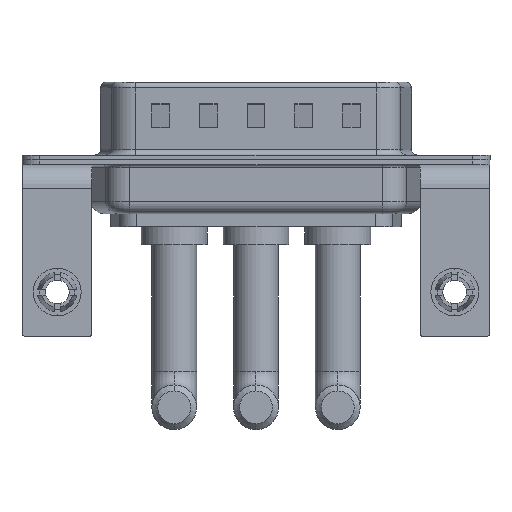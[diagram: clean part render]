
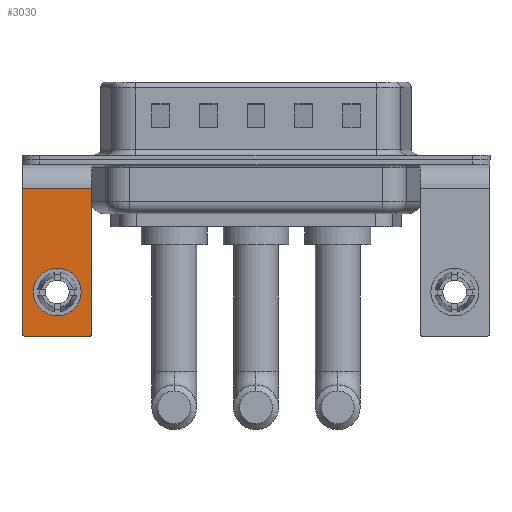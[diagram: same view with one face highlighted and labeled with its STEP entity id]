
A CAD part, front view. The second image highlights one B-rep face of the part: STEP entity #3030.
In plain terms, the highlighted planar face has unit normal (0, -1, 0).
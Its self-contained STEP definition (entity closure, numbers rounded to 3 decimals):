
#278 = EDGE_CURVE ( 'NONE', #8263, #9243, #16908, .T. ) ;
#371 = LINE ( 'NONE', #4820, #7940 ) ;
#404 = AXIS2_PLACEMENT_3D ( 'NONE', #13075, #552, #7573 ) ;
#552 = DIRECTION ( 'NONE',  ( 0., 1., 0. ) ) ;
#1110 = ORIENTED_EDGE ( 'NONE', *, *, #10544, .F. ) ;
#1682 = VERTEX_POINT ( 'NONE', #12028 ) ;
#1936 = VERTEX_POINT ( 'NONE', #9993 ) ;
#2019 = EDGE_LOOP ( 'NONE', ( #11203, #3994, #1110, #11894, #14713, #11677 ) ) ;
#2420 = EDGE_CURVE ( 'NONE', #9901, #11657, #15220, .T. ) ;
#3030 = ADVANCED_FACE ( 'NONE', ( #12803, #15634 ), #11686, .F. ) ;
#3065 = VECTOR ( 'NONE', #7328, 1000. ) ;
#3817 = EDGE_CURVE ( 'NONE', #1682, #9901, #5685, .T. ) ;
#3994 = ORIENTED_EDGE ( 'NONE', *, *, #2420, .T. ) ;
#4219 = CIRCLE ( 'NONE', #16773, 2. ) ;
#4284 = EDGE_CURVE ( 'NONE', #5242, #1682, #14102, .T. ) ;
#4475 = DIRECTION ( 'NONE',  ( 0., 0., 1. ) ) ;
#4621 = VERTEX_POINT ( 'NONE', #6673 ) ;
#4820 = CARTESIAN_POINT ( 'NONE',  ( 2.9, -6.25, -2.4 ) ) ;
#4847 = DIRECTION ( 'NONE',  ( 0., 0., 1. ) ) ;
#5165 = EDGE_CURVE ( 'NONE', #1936, #4621, #4219, .T. ) ;
#5186 = CIRCLE ( 'NONE', #11595, 2. ) ;
#5242 = VERTEX_POINT ( 'NONE', #13125 ) ;
#5439 = CARTESIAN_POINT ( 'NONE',  ( 2.9, -6.25, -14.8 ) ) ;
#5560 = AXIS2_PLACEMENT_3D ( 'NONE', #5772, #5858, #13947 ) ;
#5685 = LINE ( 'NONE', #11260, #3065 ) ;
#5772 = CARTESIAN_POINT ( 'NONE',  ( -2.65, -6.25, -14.55 ) ) ;
#5858 = DIRECTION ( 'NONE',  ( 0., -1., 0. ) ) ;
#6673 = CARTESIAN_POINT ( 'NONE',  ( 0., -6.25, -9.07 ) ) ;
#6827 = DIRECTION ( 'NONE',  ( 0., 1., 0. ) ) ;
#7141 = CARTESIAN_POINT ( 'NONE',  ( 2.9, -6.25, -14.55 ) ) ;
#7328 = DIRECTION ( 'NONE',  ( 0., 0., -1. ) ) ;
#7562 = DIRECTION ( 'NONE',  ( 0., 0., -1. ) ) ;
#7573 = DIRECTION ( 'NONE',  ( 0., 0., 1. ) ) ;
#7940 = VECTOR ( 'NONE', #7562, 1000. ) ;
#8263 = VERTEX_POINT ( 'NONE', #15278 ) ;
#8397 = EDGE_CURVE ( 'NONE', #5242, #9243, #371, .T. ) ;
#8854 = CARTESIAN_POINT ( 'NONE',  ( 0., -6.25, -11.07 ) ) ;
#9010 = AXIS2_PLACEMENT_3D ( 'NONE', #16006, #13374, #4847 ) ;
#9243 = VERTEX_POINT ( 'NONE', #7141 ) ;
#9555 = CARTESIAN_POINT ( 'NONE',  ( 0., -6.25, -11.07 ) ) ;
#9901 = VERTEX_POINT ( 'NONE', #10209 ) ;
#9993 = CARTESIAN_POINT ( 'NONE',  ( 0., -6.25, -13.07 ) ) ;
#10209 = CARTESIAN_POINT ( 'NONE',  ( -2.9, -6.25, -14.55 ) ) ;
#10544 = EDGE_CURVE ( 'NONE', #8263, #11657, #12570, .T. ) ;
#10615 = ORIENTED_EDGE ( 'NONE', *, *, #5165, .T. ) ;
#10754 = VECTOR ( 'NONE', #11234, 1000. ) ;
#10917 = VECTOR ( 'NONE', #18078, 1000. ) ;
#11203 = ORIENTED_EDGE ( 'NONE', *, *, #3817, .T. ) ;
#11234 = DIRECTION ( 'NONE',  ( -1., 0., 0. ) ) ;
#11260 = CARTESIAN_POINT ( 'NONE',  ( -2.9, -6.25, -2.4 ) ) ;
#11595 = AXIS2_PLACEMENT_3D ( 'NONE', #8854, #12978, #4475 ) ;
#11657 = VERTEX_POINT ( 'NONE', #15060 ) ;
#11677 = ORIENTED_EDGE ( 'NONE', *, *, #4284, .T. ) ;
#11686 = PLANE ( 'NONE',  #404 ) ;
#11894 = ORIENTED_EDGE ( 'NONE', *, *, #278, .T. ) ;
#12028 = CARTESIAN_POINT ( 'NONE',  ( -2.9, -6.25, -2.4 ) ) ;
#12570 = LINE ( 'NONE', #5439, #10917 ) ;
#12803 = FACE_BOUND ( 'NONE', #15481, .T. ) ;
#12978 = DIRECTION ( 'NONE',  ( 0., 1., 0. ) ) ;
#13075 = CARTESIAN_POINT ( 'NONE',  ( 2.9, -6.25, -2.4 ) ) ;
#13125 = CARTESIAN_POINT ( 'NONE',  ( 2.9, -6.25, -2.4 ) ) ;
#13374 = DIRECTION ( 'NONE',  ( 0., -1., 0. ) ) ;
#13947 = DIRECTION ( 'NONE',  ( 0., 0., 1. ) ) ;
#14102 = LINE ( 'NONE', #14280, #10754 ) ;
#14280 = CARTESIAN_POINT ( 'NONE',  ( 2.9, -6.25, -2.4 ) ) ;
#14713 = ORIENTED_EDGE ( 'NONE', *, *, #8397, .F. ) ;
#15060 = CARTESIAN_POINT ( 'NONE',  ( -2.65, -6.25, -14.8 ) ) ;
#15163 = DIRECTION ( 'NONE',  ( 0., 0., 1. ) ) ;
#15220 = CIRCLE ( 'NONE', #5560, 0.25 ) ;
#15278 = CARTESIAN_POINT ( 'NONE',  ( 2.65, -6.25, -14.8 ) ) ;
#15481 = EDGE_LOOP ( 'NONE', ( #10615, #16740 ) ) ;
#15634 = FACE_OUTER_BOUND ( 'NONE', #2019, .T. ) ;
#15675 = EDGE_CURVE ( 'NONE', #4621, #1936, #5186, .T. ) ;
#16006 = CARTESIAN_POINT ( 'NONE',  ( 2.65, -6.25, -14.55 ) ) ;
#16740 = ORIENTED_EDGE ( 'NONE', *, *, #15675, .T. ) ;
#16773 = AXIS2_PLACEMENT_3D ( 'NONE', #9555, #6827, #15163 ) ;
#16908 = CIRCLE ( 'NONE', #9010, 0.25 ) ;
#18078 = DIRECTION ( 'NONE',  ( -1., 0., 0. ) ) ;
